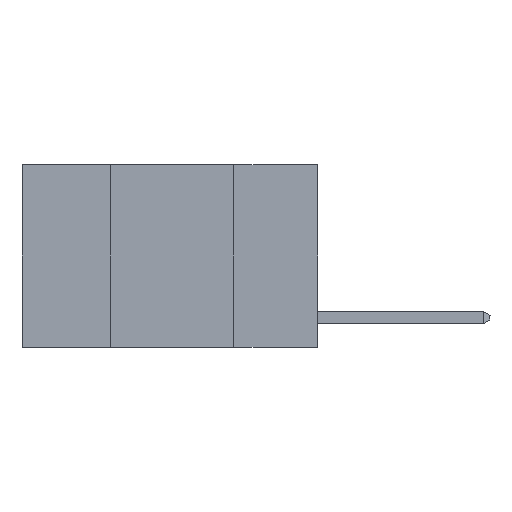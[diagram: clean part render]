
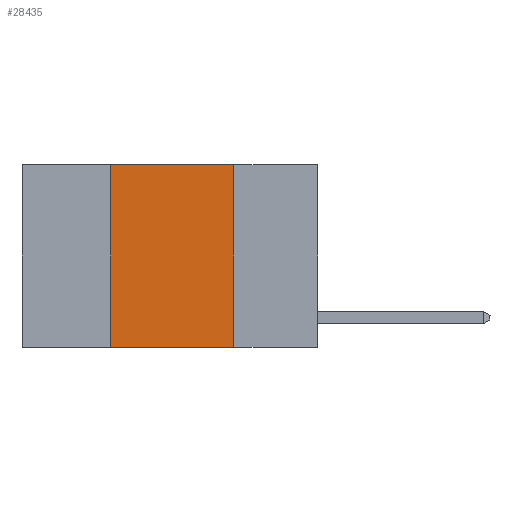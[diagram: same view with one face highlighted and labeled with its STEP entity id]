
A CAD part, left-side view. The second image highlights one B-rep face of the part: STEP entity #28435.
In plain terms, the highlighted planar face has unit normal (-1, 0, 0).
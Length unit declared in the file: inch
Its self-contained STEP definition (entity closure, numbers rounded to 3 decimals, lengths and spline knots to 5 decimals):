
#50 = ORIENTED_EDGE ( 'NONE', *, *, #14346, .F. ) ;
#752 = DIRECTION ( 'NONE',  ( 0., 0., -1. ) ) ;
#1607 = DIRECTION ( 'NONE',  ( 0., -1., 0. ) ) ;
#1730 = LINE ( 'NONE', #28277, #15142 ) ;
#2441 = EDGE_CURVE ( 'NONE', #12645, #16577, #14641, .T. ) ;
#3209 = DIRECTION ( 'NONE',  ( 1., 0., 0. ) ) ;
#3330 = VECTOR ( 'NONE', #1607, 39.37008 ) ;
#3734 = LINE ( 'NONE', #8094, #13078 ) ;
#3827 = VECTOR ( 'NONE', #5510, 39.37008 ) ;
#4133 = VERTEX_POINT ( 'NONE', #14747 ) ;
#5510 = DIRECTION ( 'NONE',  ( 0., -1., 0. ) ) ;
#6200 = DIRECTION ( 'NONE',  ( 0., 0., -1. ) ) ;
#7157 = PLANE ( 'NONE',  #26289 ) ;
#8094 = CARTESIAN_POINT ( 'NONE',  ( 0., 0.17, 0. ) ) ;
#9144 = CARTESIAN_POINT ( 'NONE',  ( 0., 0.17, 0. ) ) ;
#9414 = VERTEX_POINT ( 'NONE', #10295 ) ;
#10295 = CARTESIAN_POINT ( 'NONE',  ( 0., 0.42, -0.37 ) ) ;
#11920 = CARTESIAN_POINT ( 'NONE',  ( 0., 0.6, 0. ) ) ;
#12163 = ORIENTED_EDGE ( 'NONE', *, *, #2441, .F. ) ;
#12624 = CARTESIAN_POINT ( 'NONE',  ( 0., 0.42, 0. ) ) ;
#12645 = VERTEX_POINT ( 'NONE', #12624 ) ;
#12848 = ORIENTED_EDGE ( 'NONE', *, *, #19357, .T. ) ;
#13078 = VECTOR ( 'NONE', #6200, 39.37008 ) ;
#13189 = DIRECTION ( 'NONE',  ( 0., 0., 1. ) ) ;
#14346 = EDGE_CURVE ( 'NONE', #16577, #4133, #3734, .T. ) ;
#14641 = LINE ( 'NONE', #19283, #3827 ) ;
#14747 = CARTESIAN_POINT ( 'NONE',  ( 0., 0.17, -0.37 ) ) ;
#14802 = EDGE_LOOP ( 'NONE', ( #50, #12163, #17439, #12848 ) ) ;
#15142 = VECTOR ( 'NONE', #13189, 39.37008 ) ;
#16577 = VERTEX_POINT ( 'NONE', #9144 ) ;
#17439 = ORIENTED_EDGE ( 'NONE', *, *, #27591, .F. ) ;
#19283 = CARTESIAN_POINT ( 'NONE',  ( 0., 0.6, 0. ) ) ;
#19323 = LINE ( 'NONE', #23516, #3330 ) ;
#19357 = EDGE_CURVE ( 'NONE', #9414, #4133, #19323, .T. ) ;
#23516 = CARTESIAN_POINT ( 'NONE',  ( 0., 0.6, -0.37 ) ) ;
#24542 = FACE_OUTER_BOUND ( 'NONE', #14802, .T. ) ;
#26289 = AXIS2_PLACEMENT_3D ( 'NONE', #11920, #3209, #752 ) ;
#27591 = EDGE_CURVE ( 'NONE', #9414, #12645, #1730, .T. ) ;
#28277 = CARTESIAN_POINT ( 'NONE',  ( 0., 0.42, 0. ) ) ;
#28435 = ADVANCED_FACE ( 'NONE', ( #24542 ), #7157, .F. ) ;
